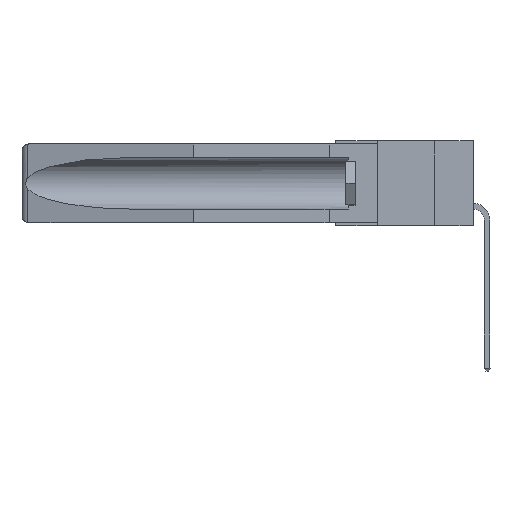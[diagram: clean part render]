
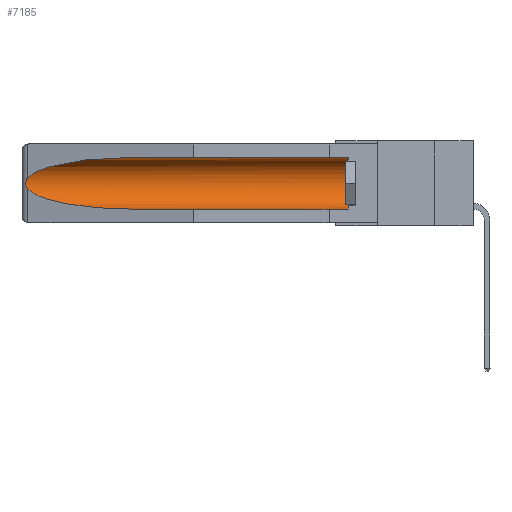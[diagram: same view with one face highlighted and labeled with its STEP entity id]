
A CAD part, left-side view. The second image highlights one B-rep face of the part: STEP entity #7185.
In plain terms, the highlighted cylindrical face has radius 2.857 mm (diameter 5.715 mm), a partial arc.
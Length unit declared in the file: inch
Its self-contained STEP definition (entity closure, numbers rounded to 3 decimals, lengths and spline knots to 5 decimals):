
#198 = CARTESIAN_POINT ( 'NONE',  ( 0.26655, 1.53094, -0.18657 ) ) ;
#490 = EDGE_CURVE ( 'NONE', #5428, #3506, #9341, .T. ) ;
#647 = EDGE_CURVE ( 'NONE', #3506, #9339, #10808, .T. ) ;
#1435 = LINE ( 'NONE', #6281, #9825 ) ;
#1727 = VERTEX_POINT ( 'NONE', #5407 ) ;
#1754 = EDGE_LOOP ( 'NONE', ( #2645, #4116, #10289, #6733, #7199, #12049 ) ) ;
#1773 = CARTESIAN_POINT ( 'NONE',  ( 0.21114, 1.30732, -0.284 ) ) ;
#1806 =( BOUNDED_CURVE ( )  B_SPLINE_CURVE ( 3, ( #8874, #2884, #7680, #11238 ),
 .UNSPECIFIED., .F., .F. ) 
 B_SPLINE_CURVE_WITH_KNOTS ( ( 4, 4 ),
 ( 4.71239, 6.08839 ),
 .UNSPECIFIED. ) 
 CURVE ( )  GEOMETRIC_REPRESENTATION_ITEM ( )  RATIONAL_B_SPLINE_CURVE ( ( 1., 0.848, 0.848, 1. ) ) 
 REPRESENTATION_ITEM ( '' )  );
#1871 = VERTEX_POINT ( 'NONE', #8166 ) ;
#2645 = ORIENTED_EDGE ( 'NONE', *, *, #11546, .T. ) ;
#2884 = CARTESIAN_POINT ( 'NONE',  ( 0.21114, 1.30732, -0.059 ) ) ;
#3506 = VERTEX_POINT ( 'NONE', #4769 ) ;
#3525 = DIRECTION ( 'NONE',  ( 0., 0., 1. ) ) ;
#4116 = ORIENTED_EDGE ( 'NONE', *, *, #13031, .T. ) ;
#4769 = CARTESIAN_POINT ( 'NONE',  ( 0.155, 0.126, -0.059 ) ) ;
#4970 = AXIS2_PLACEMENT_3D ( 'NONE', #7010, #11718, #5858 ) ;
#5190 = CARTESIAN_POINT ( 'NONE',  ( 0.26654, 1.53092, -0.15636 ) ) ;
#5371 = CARTESIAN_POINT ( 'NONE',  ( 0.26537, 1.52718, -0.19328 ) ) ;
#5407 = CARTESIAN_POINT ( 'NONE',  ( 0.26537, 1.52718, -0.14972 ) ) ;
#5428 = VERTEX_POINT ( 'NONE', #13225 ) ;
#5568 = CARTESIAN_POINT ( 'NONE',  ( 0.25451, 1.48313, -0.24835 ) ) ;
#5790 = FACE_OUTER_BOUND ( 'NONE', #1754, .T. ) ;
#5858 = DIRECTION ( 'NONE',  ( 0., 0., 1. ) ) ;
#6173 = CARTESIAN_POINT ( 'NONE',  ( 0.2675, 1.53308, -0.17534 ) ) ;
#6281 = CARTESIAN_POINT ( 'NONE',  ( 0.155, -0.30754, -0.284 ) ) ;
#6350 = CARTESIAN_POINT ( 'NONE',  ( 0.155, 1.07973, -0.059 ) ) ;
#6376 = CARTESIAN_POINT ( 'NONE',  ( 0.2675, 1.53308, -0.16763 ) ) ;
#6733 = ORIENTED_EDGE ( 'NONE', *, *, #13336, .F. ) ;
#7010 = CARTESIAN_POINT ( 'NONE',  ( 0.155, 0.126, -0.1715 ) ) ;
#7185 = ADVANCED_FACE ( 'NONE', ( #5790 ), #8754, .F. ) ;
#7199 = ORIENTED_EDGE ( 'NONE', *, *, #490, .T. ) ;
#7680 = CARTESIAN_POINT ( 'NONE',  ( 0.25451, 1.48313, -0.09465 ) ) ;
#8166 = CARTESIAN_POINT ( 'NONE',  ( 0.155, 1.07973, -0.284 ) ) ;
#8305 = B_SPLINE_CURVE_WITH_KNOTS ( 'NONE', 3,
 ( #13425, #12325, #5190, #13528, #6376, #6173, #14527, #198, #8539, #11180 ),
 .UNSPECIFIED., .F., .F.,
 ( 4, 2, 2, 2, 4 ),
 ( 0., 0.00029, 0.00058, 0.00087, 0.00117 ),
 .UNSPECIFIED. ) ;
#8347 = DIRECTION ( 'NONE',  ( 0., 1., 0. ) ) ;
#8375 = CARTESIAN_POINT ( 'NONE',  ( 0.26537, 1.52718, -0.19328 ) ) ;
#8539 = CARTESIAN_POINT ( 'NONE',  ( 0.26597, 1.5296, -0.19026 ) ) ;
#8754 = CYLINDRICAL_SURFACE ( 'NONE', #13253, 0.1125 ) ;
#8874 = CARTESIAN_POINT ( 'NONE',  ( 0.155, 1.07973, -0.059 ) ) ;
#9339 = VERTEX_POINT ( 'NONE', #6350 ) ;
#9341 = CIRCLE ( 'NONE', #4970, 0.1125 ) ;
#9514 = CARTESIAN_POINT ( 'NONE',  ( 0.155, -0.30754, -0.1715 ) ) ;
#9825 = VECTOR ( 'NONE', #9866, 39.37008 ) ;
#9866 = DIRECTION ( 'NONE',  ( 0., 1., 0. ) ) ;
#9872 = EDGE_CURVE ( 'NONE', #12805, #1871, #10896, .T. ) ;
#10124 = CARTESIAN_POINT ( 'NONE',  ( 0.155, 1.07973, -0.284 ) ) ;
#10289 = ORIENTED_EDGE ( 'NONE', *, *, #9872, .T. ) ;
#10808 = LINE ( 'NONE', #13006, #11195 ) ;
#10896 =( BOUNDED_CURVE ( )  B_SPLINE_CURVE ( 3, ( #5371, #5568, #1773, #10124 ),
 .UNSPECIFIED., .F., .F. ) 
 B_SPLINE_CURVE_WITH_KNOTS ( ( 4, 4 ),
 ( 0.1948, 1.5708 ),
 .UNSPECIFIED. ) 
 CURVE ( )  GEOMETRIC_REPRESENTATION_ITEM ( )  RATIONAL_B_SPLINE_CURVE ( ( 1., 0.848, 0.848, 1. ) ) 
 REPRESENTATION_ITEM ( '' )  );
#11180 = CARTESIAN_POINT ( 'NONE',  ( 0.26537, 1.52718, -0.19328 ) ) ;
#11195 = VECTOR ( 'NONE', #14320, 39.37008 ) ;
#11238 = CARTESIAN_POINT ( 'NONE',  ( 0.26537, 1.52718, -0.14972 ) ) ;
#11546 = EDGE_CURVE ( 'NONE', #9339, #1727, #1806, .T. ) ;
#11718 = DIRECTION ( 'NONE',  ( 0., -1., 0. ) ) ;
#12049 = ORIENTED_EDGE ( 'NONE', *, *, #647, .T. ) ;
#12325 = CARTESIAN_POINT ( 'NONE',  ( 0.26597, 1.52961, -0.15275 ) ) ;
#12805 = VERTEX_POINT ( 'NONE', #8375 ) ;
#13006 = CARTESIAN_POINT ( 'NONE',  ( 0.155, -0.30754, -0.059 ) ) ;
#13031 = EDGE_CURVE ( 'NONE', #1727, #12805, #8305, .T. ) ;
#13225 = CARTESIAN_POINT ( 'NONE',  ( 0.155, 0.126, -0.284 ) ) ;
#13253 = AXIS2_PLACEMENT_3D ( 'NONE', #9514, #8347, #3525 ) ;
#13336 = EDGE_CURVE ( 'NONE', #5428, #1871, #1435, .T. ) ;
#13425 = CARTESIAN_POINT ( 'NONE',  ( 0.26537, 1.52718, -0.14972 ) ) ;
#13528 = CARTESIAN_POINT ( 'NONE',  ( 0.2673, 1.5327, -0.16383 ) ) ;
#14320 = DIRECTION ( 'NONE',  ( 0., 1., 0. ) ) ;
#14527 = CARTESIAN_POINT ( 'NONE',  ( 0.2673, 1.53269, -0.17917 ) ) ;
